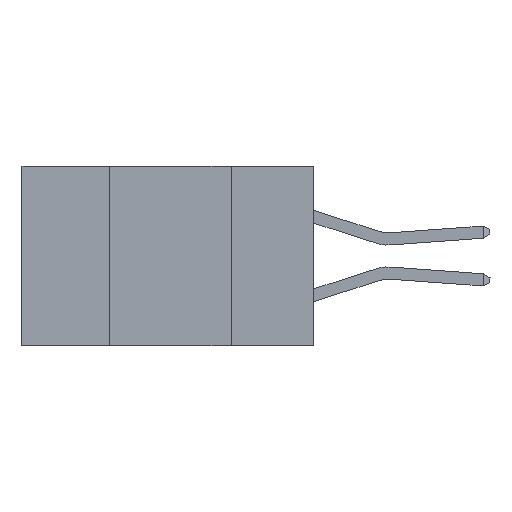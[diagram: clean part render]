
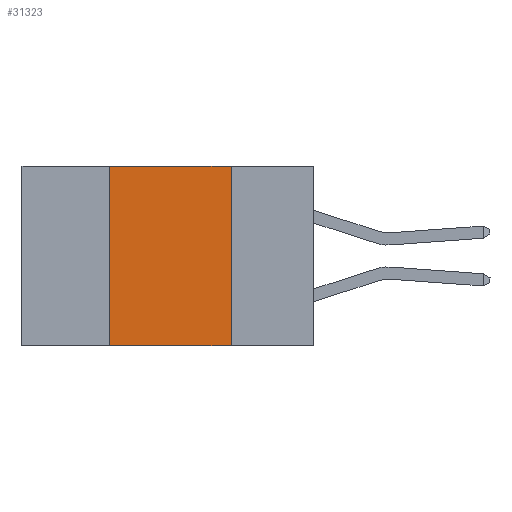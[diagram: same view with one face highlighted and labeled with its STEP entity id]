
A CAD part, left-side view. The second image highlights one B-rep face of the part: STEP entity #31323.
In plain terms, the highlighted planar face has unit normal (-1, 0, 0).
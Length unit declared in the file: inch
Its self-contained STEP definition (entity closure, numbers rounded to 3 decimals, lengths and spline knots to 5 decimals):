
#512 = DIRECTION ( 'NONE',  ( 0., 0., 1. ) ) ;
#2424 = CARTESIAN_POINT ( 'NONE',  ( 0., 0.42, 0. ) ) ;
#3055 = ORIENTED_EDGE ( 'NONE', *, *, #19246, .F. ) ;
#5091 = LINE ( 'NONE', #27193, #18410 ) ;
#5350 = ORIENTED_EDGE ( 'NONE', *, *, #19689, .F. ) ;
#6514 = VECTOR ( 'NONE', #16286, 39.37008 ) ;
#7895 = VECTOR ( 'NONE', #9401, 39.37008 ) ;
#8564 = VERTEX_POINT ( 'NONE', #26777 ) ;
#8742 = ORIENTED_EDGE ( 'NONE', *, *, #13211, .T. ) ;
#9031 = PLANE ( 'NONE',  #14006 ) ;
#9070 = CARTESIAN_POINT ( 'NONE',  ( 0., 0.6, 0. ) ) ;
#9155 = CARTESIAN_POINT ( 'NONE',  ( 0., 0.17, 0. ) ) ;
#9401 = DIRECTION ( 'NONE',  ( 0., -1., 0. ) ) ;
#12774 = VECTOR ( 'NONE', #512, 39.37008 ) ;
#13211 = EDGE_CURVE ( 'NONE', #30998, #8564, #13834, .T. ) ;
#13834 = LINE ( 'NONE', #23811, #7895 ) ;
#14006 = AXIS2_PLACEMENT_3D ( 'NONE', #16886, #26393, #18868 ) ;
#14313 = LINE ( 'NONE', #9070, #6514 ) ;
#16286 = DIRECTION ( 'NONE',  ( 0., -1., 0. ) ) ;
#16886 = CARTESIAN_POINT ( 'NONE',  ( 0., 0.6, 0. ) ) ;
#18410 = VECTOR ( 'NONE', #32252, 39.37008 ) ;
#18868 = DIRECTION ( 'NONE',  ( 0., 0., -1. ) ) ;
#19246 = EDGE_CURVE ( 'NONE', #30998, #26679, #25706, .T. ) ;
#19348 = FACE_OUTER_BOUND ( 'NONE', #29647, .T. ) ;
#19689 = EDGE_CURVE ( 'NONE', #26679, #31866, #14313, .T. ) ;
#20377 = EDGE_CURVE ( 'NONE', #31866, #8564, #5091, .T. ) ;
#21672 = CARTESIAN_POINT ( 'NONE',  ( 0., 0.42, -0.37 ) ) ;
#22923 = CARTESIAN_POINT ( 'NONE',  ( 0., 0.42, 0. ) ) ;
#23811 = CARTESIAN_POINT ( 'NONE',  ( 0., 0.6, -0.37 ) ) ;
#25706 = LINE ( 'NONE', #22923, #12774 ) ;
#26393 = DIRECTION ( 'NONE',  ( 1., 0., 0. ) ) ;
#26679 = VERTEX_POINT ( 'NONE', #2424 ) ;
#26777 = CARTESIAN_POINT ( 'NONE',  ( 0., 0.17, -0.37 ) ) ;
#26954 = ORIENTED_EDGE ( 'NONE', *, *, #20377, .F. ) ;
#27193 = CARTESIAN_POINT ( 'NONE',  ( 0., 0.17, 0. ) ) ;
#29647 = EDGE_LOOP ( 'NONE', ( #26954, #5350, #3055, #8742 ) ) ;
#30998 = VERTEX_POINT ( 'NONE', #21672 ) ;
#31323 = ADVANCED_FACE ( 'NONE', ( #19348 ), #9031, .F. ) ;
#31866 = VERTEX_POINT ( 'NONE', #9155 ) ;
#32252 = DIRECTION ( 'NONE',  ( 0., 0., -1. ) ) ;
